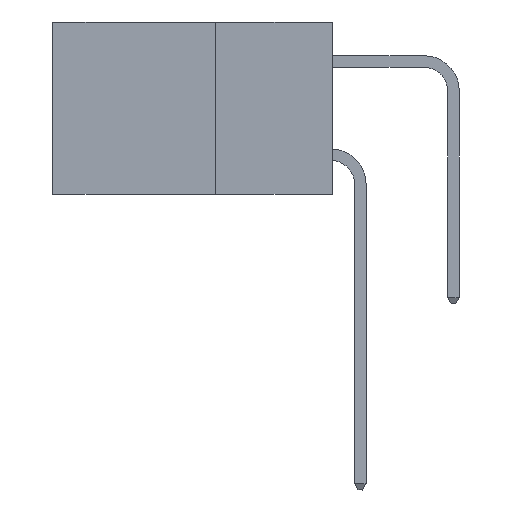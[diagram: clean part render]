
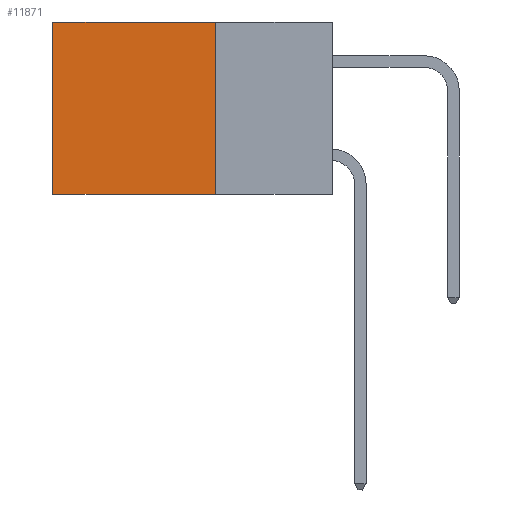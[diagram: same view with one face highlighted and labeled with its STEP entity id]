
A CAD part, left-side view. The second image highlights one B-rep face of the part: STEP entity #11871.
In plain terms, the highlighted planar face has unit normal (-1, 0, 0).
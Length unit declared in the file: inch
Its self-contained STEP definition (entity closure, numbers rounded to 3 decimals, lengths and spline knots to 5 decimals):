
#180 = VECTOR ( 'NONE', #14025, 39.37008 ) ;
#730 = ORIENTED_EDGE ( 'NONE', *, *, #14621, .F. ) ;
#846 = EDGE_CURVE ( 'NONE', #15831, #10674, #13321, .T. ) ;
#932 = CARTESIAN_POINT ( 'NONE',  ( 0.298, 0.25, 0. ) ) ;
#2875 = ORIENTED_EDGE ( 'NONE', *, *, #9536, .F. ) ;
#2977 = PLANE ( 'NONE',  #5564 ) ;
#3090 = FACE_OUTER_BOUND ( 'NONE', #13497, .T. ) ;
#4271 = VECTOR ( 'NONE', #9990, 39.37008 ) ;
#4462 = VECTOR ( 'NONE', #5071, 39.37008 ) ;
#4556 = CARTESIAN_POINT ( 'NONE',  ( 0.298, 0.25, 0. ) ) ;
#5071 = DIRECTION ( 'NONE',  ( 0., 0., -1. ) ) ;
#5564 = AXIS2_PLACEMENT_3D ( 'NONE', #12802, #7248, #10060 ) ;
#7248 = DIRECTION ( 'NONE',  ( 1., 0., 0. ) ) ;
#7399 = CARTESIAN_POINT ( 'NONE',  ( 0.298, 0.6, 0. ) ) ;
#8720 = EDGE_CURVE ( 'NONE', #10674, #17331, #9953, .T. ) ;
#9536 = EDGE_CURVE ( 'NONE', #15831, #16537, #9936, .T. ) ;
#9936 = LINE ( 'NONE', #17849, #4462 ) ;
#9953 = LINE ( 'NONE', #13854, #4271 ) ;
#9990 = DIRECTION ( 'NONE',  ( 0., 0., -1. ) ) ;
#10060 = DIRECTION ( 'NONE',  ( 0., 0., -1. ) ) ;
#10674 = VERTEX_POINT ( 'NONE', #7399 ) ;
#11871 = ADVANCED_FACE ( 'NONE', ( #3090 ), #2977, .F. ) ;
#12415 = ORIENTED_EDGE ( 'NONE', *, *, #846, .T. ) ;
#12673 = VECTOR ( 'NONE', #14242, 39.37008 ) ;
#12802 = CARTESIAN_POINT ( 'NONE',  ( 0.298, 0.25, 0. ) ) ;
#13321 = LINE ( 'NONE', #932, #12673 ) ;
#13497 = EDGE_LOOP ( 'NONE', ( #17384, #730, #2875, #12415 ) ) ;
#13854 = CARTESIAN_POINT ( 'NONE',  ( 0.298, 0.6, 0. ) ) ;
#14025 = DIRECTION ( 'NONE',  ( 0., 1., 0. ) ) ;
#14242 = DIRECTION ( 'NONE',  ( 0., 1., 0. ) ) ;
#14378 = LINE ( 'NONE', #16846, #180 ) ;
#14621 = EDGE_CURVE ( 'NONE', #16537, #17331, #14378, .T. ) ;
#15002 = CARTESIAN_POINT ( 'NONE',  ( 0.298, 0.6, -0.37 ) ) ;
#15831 = VERTEX_POINT ( 'NONE', #4556 ) ;
#16537 = VERTEX_POINT ( 'NONE', #16981 ) ;
#16846 = CARTESIAN_POINT ( 'NONE',  ( 0.298, 0.25, -0.37 ) ) ;
#16981 = CARTESIAN_POINT ( 'NONE',  ( 0.298, 0.25, -0.37 ) ) ;
#17331 = VERTEX_POINT ( 'NONE', #15002 ) ;
#17384 = ORIENTED_EDGE ( 'NONE', *, *, #8720, .T. ) ;
#17849 = CARTESIAN_POINT ( 'NONE',  ( 0.298, 0.25, 0. ) ) ;
